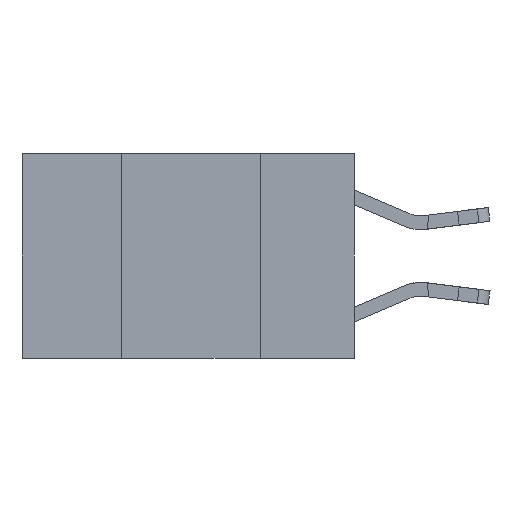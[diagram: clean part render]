
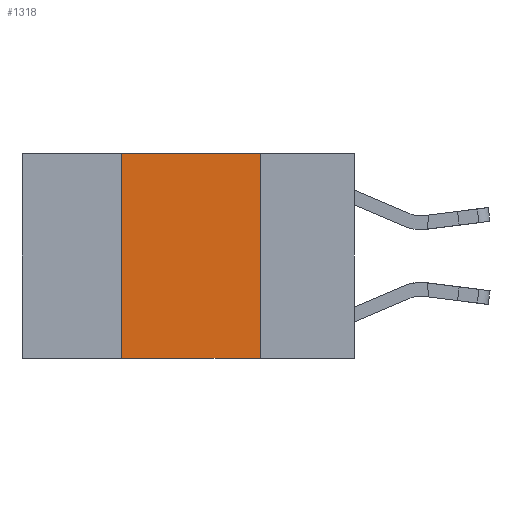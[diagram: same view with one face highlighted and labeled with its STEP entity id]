
A CAD part, left-side view. The second image highlights one B-rep face of the part: STEP entity #1318.
In plain terms, the highlighted planar face has unit normal (-1, 0, 0).
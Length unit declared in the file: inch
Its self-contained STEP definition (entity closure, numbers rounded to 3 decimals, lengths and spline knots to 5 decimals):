
#26 = ORIENTED_EDGE ( 'NONE', *, *, #5795, .F. ) ;
#1318 = ADVANCED_FACE ( 'NONE', ( #22616 ), #1627, .F. ) ;
#1513 = CARTESIAN_POINT ( 'NONE',  ( 0., 0.6, -0.37 ) ) ;
#1563 = DIRECTION ( 'NONE',  ( 0., 0., -1. ) ) ;
#1595 = DIRECTION ( 'NONE',  ( 1., 0., 0. ) ) ;
#1627 = PLANE ( 'NONE',  #17110 ) ;
#1728 = DIRECTION ( 'NONE',  ( 0., 0., -1. ) ) ;
#1938 = CARTESIAN_POINT ( 'NONE',  ( 0., 0.6, 0. ) ) ;
#2273 = LINE ( 'NONE', #1513, #15850 ) ;
#3340 = CARTESIAN_POINT ( 'NONE',  ( 0., 0.42, 0. ) ) ;
#3492 = CARTESIAN_POINT ( 'NONE',  ( 0., 0.42, 0. ) ) ;
#3810 = CARTESIAN_POINT ( 'NONE',  ( 0., 0.17, 0. ) ) ;
#4598 = VECTOR ( 'NONE', #8769, 39.37008 ) ;
#5080 = EDGE_CURVE ( 'NONE', #16708, #16170, #2273, .T. ) ;
#5795 = EDGE_CURVE ( 'NONE', #16708, #13210, #18983, .T. ) ;
#5835 = EDGE_CURVE ( 'NONE', #13210, #18061, #21867, .T. ) ;
#6339 = EDGE_LOOP ( 'NONE', ( #21212, #12928, #26, #21979 ) ) ;
#7613 = VECTOR ( 'NONE', #1728, 39.37008 ) ;
#8769 = DIRECTION ( 'NONE',  ( 0., 0., 1. ) ) ;
#8838 = DIRECTION ( 'NONE',  ( 0., -1., 0. ) ) ;
#10482 = CARTESIAN_POINT ( 'NONE',  ( 0., 0.6, 0. ) ) ;
#12928 = ORIENTED_EDGE ( 'NONE', *, *, #5835, .F. ) ;
#13210 = VERTEX_POINT ( 'NONE', #3492 ) ;
#15020 = CARTESIAN_POINT ( 'NONE',  ( 0., 0.42, -0.37 ) ) ;
#15651 = DIRECTION ( 'NONE',  ( 0., -1., 0. ) ) ;
#15847 = CARTESIAN_POINT ( 'NONE',  ( 0., 0.17, 0. ) ) ;
#15850 = VECTOR ( 'NONE', #15651, 39.37008 ) ;
#16170 = VERTEX_POINT ( 'NONE', #22113 ) ;
#16708 = VERTEX_POINT ( 'NONE', #15020 ) ;
#16827 = LINE ( 'NONE', #15847, #7613 ) ;
#17110 = AXIS2_PLACEMENT_3D ( 'NONE', #1938, #1595, #1563 ) ;
#17419 = VECTOR ( 'NONE', #8838, 39.37008 ) ;
#18061 = VERTEX_POINT ( 'NONE', #3810 ) ;
#18983 = LINE ( 'NONE', #3340, #4598 ) ;
#21212 = ORIENTED_EDGE ( 'NONE', *, *, #21509, .F. ) ;
#21509 = EDGE_CURVE ( 'NONE', #18061, #16170, #16827, .T. ) ;
#21867 = LINE ( 'NONE', #10482, #17419 ) ;
#21979 = ORIENTED_EDGE ( 'NONE', *, *, #5080, .T. ) ;
#22113 = CARTESIAN_POINT ( 'NONE',  ( 0., 0.17, -0.37 ) ) ;
#22616 = FACE_OUTER_BOUND ( 'NONE', #6339, .T. ) ;
